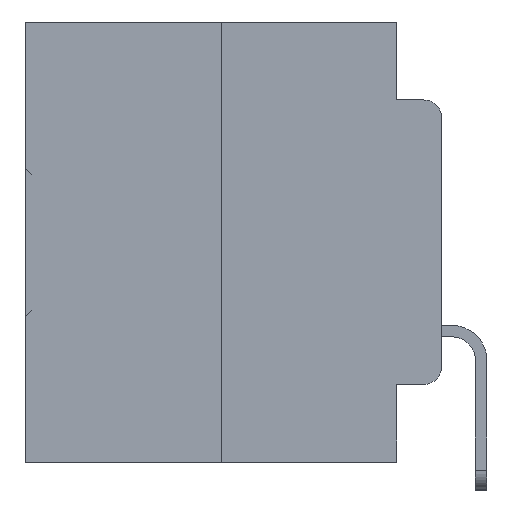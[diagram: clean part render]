
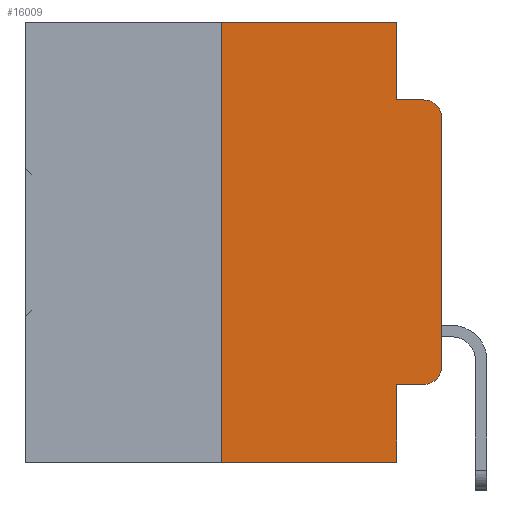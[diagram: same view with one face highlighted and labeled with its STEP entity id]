
A CAD part, left-side view. The second image highlights one B-rep face of the part: STEP entity #16009.
In plain terms, the highlighted planar face has unit normal (-1, 0, 0).
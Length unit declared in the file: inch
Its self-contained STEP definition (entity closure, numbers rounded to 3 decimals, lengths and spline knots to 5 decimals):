
#402 = VERTEX_POINT ( 'NONE', #7201 ) ;
#775 = CARTESIAN_POINT ( 'NONE',  ( 0., 0.051, -0.5 ) ) ;
#1093 = VECTOR ( 'NONE', #4903, 39.37008 ) ;
#1164 = LINE ( 'NONE', #4061, #21021 ) ;
#1304 = EDGE_CURVE ( 'NONE', #402, #12730, #22576, .T. ) ;
#1506 = CARTESIAN_POINT ( 'NONE',  ( 0., 0.02, -0.1085 ) ) ;
#3140 = EDGE_CURVE ( 'NONE', #402, #28754, #16685, .T. ) ;
#3542 = DIRECTION ( 'NONE',  ( 0., 0., 1. ) ) ;
#4061 = CARTESIAN_POINT ( 'NONE',  ( 0., 0.051, 0. ) ) ;
#4295 = DIRECTION ( 'NONE',  ( 0., 0., -1. ) ) ;
#4454 = ORIENTED_EDGE ( 'NONE', *, *, #10524, .F. ) ;
#4780 = ORIENTED_EDGE ( 'NONE', *, *, #5015, .F. ) ;
#4903 = DIRECTION ( 'NONE',  ( 0., -1., 0. ) ) ;
#4986 = ORIENTED_EDGE ( 'NONE', *, *, #3140, .F. ) ;
#5015 = EDGE_CURVE ( 'NONE', #15027, #16841, #18089, .T. ) ;
#5600 = LINE ( 'NONE', #22352, #12017 ) ;
#5636 = CARTESIAN_POINT ( 'NONE',  ( 0., 0., 0. ) ) ;
#5831 = CARTESIAN_POINT ( 'NONE',  ( 0., 0.051, -0.0885 ) ) ;
#6070 = AXIS2_PLACEMENT_3D ( 'NONE', #14386, #32509, #17061 ) ;
#6803 = EDGE_CURVE ( 'NONE', #15027, #28754, #8372, .T. ) ;
#6921 = CARTESIAN_POINT ( 'NONE',  ( 0., 0., -0.1085 ) ) ;
#6934 = EDGE_LOOP ( 'NONE', ( #17437, #10949, #7584, #4454, #27578, #4780, #28077, #4986, #23957, #6973 ) ) ;
#6973 = ORIENTED_EDGE ( 'NONE', *, *, #30477, .T. ) ;
#7201 = CARTESIAN_POINT ( 'NONE',  ( 0., 0.051, -0.4115 ) ) ;
#7584 = ORIENTED_EDGE ( 'NONE', *, *, #12359, .F. ) ;
#7704 = CARTESIAN_POINT ( 'NONE',  ( 0., 0.051, -0.4115 ) ) ;
#7728 = CARTESIAN_POINT ( 'NONE',  ( 0., 0.25, -0.5 ) ) ;
#8372 = LINE ( 'NONE', #31981, #27728 ) ;
#9562 = VECTOR ( 'NONE', #33982, 39.37008 ) ;
#9982 = CARTESIAN_POINT ( 'NONE',  ( 0., 0.02, -0.0885 ) ) ;
#10243 = VERTEX_POINT ( 'NONE', #11067 ) ;
#10382 = VERTEX_POINT ( 'NONE', #22122 ) ;
#10524 = EDGE_CURVE ( 'NONE', #10243, #28219, #1164, .T. ) ;
#10949 = ORIENTED_EDGE ( 'NONE', *, *, #15925, .T. ) ;
#11067 = CARTESIAN_POINT ( 'NONE',  ( 0., 0.051, 0. ) ) ;
#12017 = VECTOR ( 'NONE', #32554, 39.37008 ) ;
#12359 = EDGE_CURVE ( 'NONE', #28219, #18578, #5600, .T. ) ;
#12431 = VECTOR ( 'NONE', #18254, 39.37008 ) ;
#12730 = VERTEX_POINT ( 'NONE', #28974 ) ;
#12808 = DIRECTION ( 'NONE',  ( 1., 0., 0. ) ) ;
#13744 = VECTOR ( 'NONE', #24266, 39.37008 ) ;
#14386 = CARTESIAN_POINT ( 'NONE',  ( 0., 0.02, -0.3915 ) ) ;
#15027 = VERTEX_POINT ( 'NONE', #7728 ) ;
#15925 = EDGE_CURVE ( 'NONE', #21864, #18578, #31350, .T. ) ;
#15939 = CARTESIAN_POINT ( 'NONE',  ( 0., 0.051, 0. ) ) ;
#16009 = ADVANCED_FACE ( 'NONE', ( #28151 ), #23233, .F. ) ;
#16522 = DIRECTION ( 'NONE',  ( 0., -1., 0. ) ) ;
#16685 = LINE ( 'NONE', #15939, #9562 ) ;
#16841 = VERTEX_POINT ( 'NONE', #26771 ) ;
#17061 = DIRECTION ( 'NONE',  ( 0., 0., -1. ) ) ;
#17437 = ORIENTED_EDGE ( 'NONE', *, *, #19463, .T. ) ;
#17592 = AXIS2_PLACEMENT_3D ( 'NONE', #28409, #12808, #30984 ) ;
#18089 = LINE ( 'NONE', #19725, #24176 ) ;
#18254 = DIRECTION ( 'NONE',  ( 0., -1., 0. ) ) ;
#18578 = VERTEX_POINT ( 'NONE', #9982 ) ;
#19463 = EDGE_CURVE ( 'NONE', #10382, #21864, #33595, .T. ) ;
#19725 = CARTESIAN_POINT ( 'NONE',  ( 0., 0.25, 0. ) ) ;
#20298 = LINE ( 'NONE', #31112, #12431 ) ;
#20424 = DIRECTION ( 'NONE',  ( -1., 0., 0. ) ) ;
#21021 = VECTOR ( 'NONE', #27978, 39.37008 ) ;
#21864 = VERTEX_POINT ( 'NONE', #6921 ) ;
#22122 = CARTESIAN_POINT ( 'NONE',  ( 0., 0., -0.3915 ) ) ;
#22352 = CARTESIAN_POINT ( 'NONE',  ( 0., 0.051, -0.0885 ) ) ;
#22576 = LINE ( 'NONE', #7704, #1093 ) ;
#22624 = EDGE_CURVE ( 'NONE', #16841, #10243, #20298, .T. ) ;
#23233 = PLANE ( 'NONE',  #17592 ) ;
#23957 = ORIENTED_EDGE ( 'NONE', *, *, #1304, .T. ) ;
#24176 = VECTOR ( 'NONE', #3542, 39.37008 ) ;
#24266 = DIRECTION ( 'NONE',  ( 0., 0., 1. ) ) ;
#26771 = CARTESIAN_POINT ( 'NONE',  ( 0., 0.25, 0. ) ) ;
#27578 = ORIENTED_EDGE ( 'NONE', *, *, #22624, .F. ) ;
#27728 = VECTOR ( 'NONE', #16522, 39.37008 ) ;
#27978 = DIRECTION ( 'NONE',  ( 0., 0., -1. ) ) ;
#28077 = ORIENTED_EDGE ( 'NONE', *, *, #6803, .T. ) ;
#28151 = FACE_OUTER_BOUND ( 'NONE', #6934, .T. ) ;
#28219 = VERTEX_POINT ( 'NONE', #5831 ) ;
#28343 = CIRCLE ( 'NONE', #6070, 0.02 ) ;
#28409 = CARTESIAN_POINT ( 'NONE',  ( 0., 0.473, 0. ) ) ;
#28754 = VERTEX_POINT ( 'NONE', #775 ) ;
#28974 = CARTESIAN_POINT ( 'NONE',  ( 0., 0.02, -0.4115 ) ) ;
#30477 = EDGE_CURVE ( 'NONE', #12730, #10382, #28343, .T. ) ;
#30984 = DIRECTION ( 'NONE',  ( 0., 0., -1. ) ) ;
#31112 = CARTESIAN_POINT ( 'NONE',  ( 0., 0.473, 0. ) ) ;
#31350 = CIRCLE ( 'NONE', #33749, 0.02 ) ;
#31981 = CARTESIAN_POINT ( 'NONE',  ( 0., 0.473, -0.5 ) ) ;
#32509 = DIRECTION ( 'NONE',  ( -1., 0., 0. ) ) ;
#32554 = DIRECTION ( 'NONE',  ( 0., -1., 0. ) ) ;
#33595 = LINE ( 'NONE', #5636, #13744 ) ;
#33749 = AXIS2_PLACEMENT_3D ( 'NONE', #1506, #20424, #4295 ) ;
#33982 = DIRECTION ( 'NONE',  ( 0., 0., -1. ) ) ;
